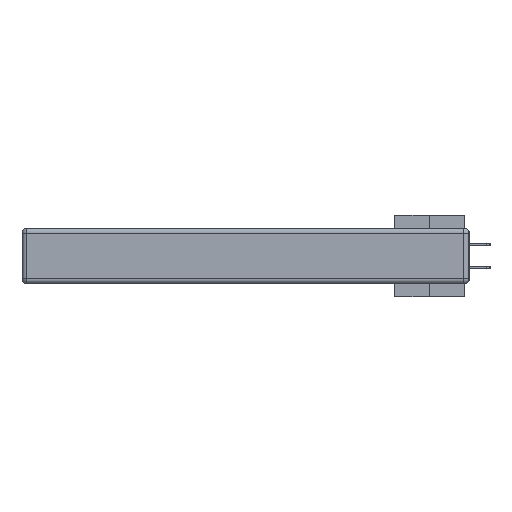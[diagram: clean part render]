
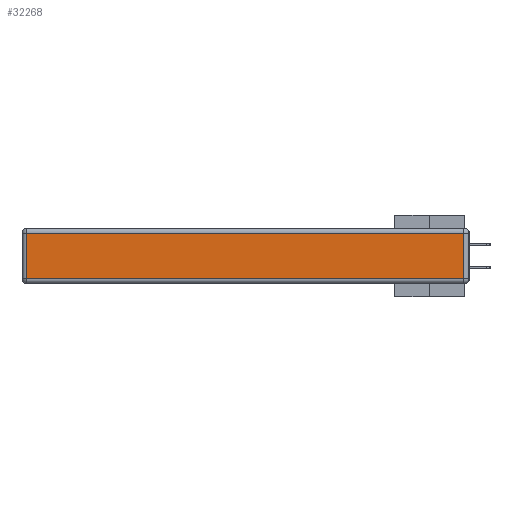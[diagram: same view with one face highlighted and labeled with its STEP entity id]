
A CAD part, left-side view. The second image highlights one B-rep face of the part: STEP entity #32268.
In plain terms, the highlighted planar face has unit normal (-1, 0, 0).
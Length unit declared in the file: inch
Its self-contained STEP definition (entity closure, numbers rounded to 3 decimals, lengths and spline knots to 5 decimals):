
#411 = EDGE_CURVE ( 'NONE', #7001, #20706, #23552, .T. ) ;
#1241 = ORIENTED_EDGE ( 'NONE', *, *, #29003, .T. ) ;
#2246 = EDGE_CURVE ( 'NONE', #35072, #7001, #13703, .T. ) ;
#2282 = DIRECTION ( 'NONE',  ( 0., 1., 0. ) ) ;
#4423 = PLANE ( 'NONE',  #29774 ) ;
#4553 = DIRECTION ( 'NONE',  ( -1., 0., 0. ) ) ;
#4573 = EDGE_CURVE ( 'NONE', #20706, #8297, #37435, .T. ) ;
#6828 = VECTOR ( 'NONE', #21040, 39.37008 ) ;
#7001 = VERTEX_POINT ( 'NONE', #31104 ) ;
#8297 = VERTEX_POINT ( 'NONE', #19177 ) ;
#10449 = CARTESIAN_POINT ( 'NONE',  ( 0., 0.03, -0.313 ) ) ;
#13703 = LINE ( 'NONE', #32467, #6828 ) ;
#13750 = EDGE_LOOP ( 'NONE', ( #35378, #23405, #1241, #26721 ) ) ;
#14526 = CARTESIAN_POINT ( 'NONE',  ( 0., 0.03, -0.343 ) ) ;
#17219 = CARTESIAN_POINT ( 'NONE',  ( 0., 0., -0.343 ) ) ;
#19019 = LINE ( 'NONE', #21235, #19522 ) ;
#19177 = CARTESIAN_POINT ( 'NONE',  ( 0., 0.03, -0.03 ) ) ;
#19522 = VECTOR ( 'NONE', #2282, 39.37008 ) ;
#20706 = VERTEX_POINT ( 'NONE', #10449 ) ;
#20987 = CARTESIAN_POINT ( 'NONE',  ( 0., 2.72, -0.03 ) ) ;
#21040 = DIRECTION ( 'NONE',  ( 0., 0., -1. ) ) ;
#21235 = CARTESIAN_POINT ( 'NONE',  ( 0., 2.75, -0.03 ) ) ;
#22628 = FACE_OUTER_BOUND ( 'NONE', #13750, .T. ) ;
#23405 = ORIENTED_EDGE ( 'NONE', *, *, #4573, .T. ) ;
#23552 = LINE ( 'NONE', #25858, #32828 ) ;
#25858 = CARTESIAN_POINT ( 'NONE',  ( 0., 0., -0.313 ) ) ;
#26471 = DIRECTION ( 'NONE',  ( 0., 0., 1. ) ) ;
#26606 = DIRECTION ( 'NONE',  ( 0., 0., 1. ) ) ;
#26721 = ORIENTED_EDGE ( 'NONE', *, *, #2246, .T. ) ;
#29003 = EDGE_CURVE ( 'NONE', #8297, #35072, #19019, .T. ) ;
#29127 = VECTOR ( 'NONE', #26606, 39.37008 ) ;
#29774 = AXIS2_PLACEMENT_3D ( 'NONE', #17219, #4553, #26471 ) ;
#31104 = CARTESIAN_POINT ( 'NONE',  ( 0., 2.72, -0.313 ) ) ;
#32268 = ADVANCED_FACE ( 'NONE', ( #22628 ), #4423, .T. ) ;
#32467 = CARTESIAN_POINT ( 'NONE',  ( 0., 2.72, -0.343 ) ) ;
#32828 = VECTOR ( 'NONE', #34861, 39.37008 ) ;
#34861 = DIRECTION ( 'NONE',  ( 0., -1., 0. ) ) ;
#35072 = VERTEX_POINT ( 'NONE', #20987 ) ;
#35378 = ORIENTED_EDGE ( 'NONE', *, *, #411, .T. ) ;
#37435 = LINE ( 'NONE', #14526, #29127 ) ;
